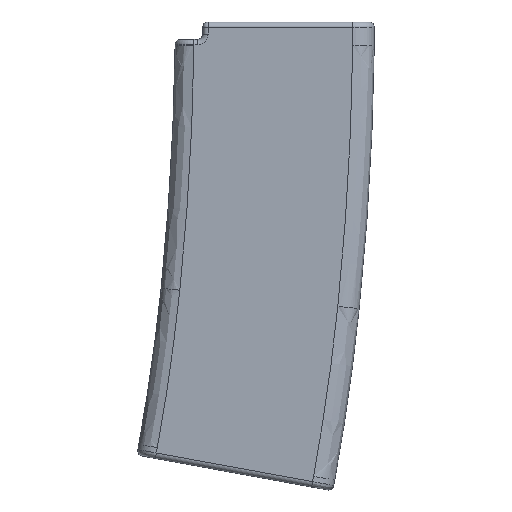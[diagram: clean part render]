
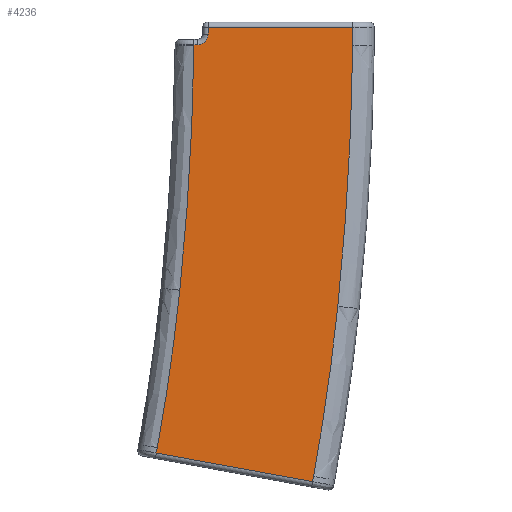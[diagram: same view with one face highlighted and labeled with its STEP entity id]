
A CAD part, top view. The second image highlights one B-rep face of the part: STEP entity #4236.
In plain terms, the highlighted planar face has unit normal (0, 0, 1).
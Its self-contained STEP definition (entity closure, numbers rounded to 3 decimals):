
#112=PLANE('',#4756);
#263=LINE('',#8074,#506);
#296=LINE('',#8319,#539);
#298=LINE('',#8379,#541);
#300=LINE('',#8392,#543);
#302=LINE('',#8400,#545);
#321=LINE('',#8475,#564);
#349=LINE('',#9411,#592);
#352=LINE('',#9417,#595);
#506=VECTOR('',#5561,10.);
#539=VECTOR('',#5660,10.);
#541=VECTOR('',#5662,10.);
#543=VECTOR('',#5678,10.);
#545=VECTOR('',#5686,10.);
#564=VECTOR('',#5777,10.);
#592=VECTOR('',#5985,10.);
#595=VECTOR('',#5994,10.);
#1068=FACE_OUTER_BOUND('',#1337,.T.);
#1337=EDGE_LOOP('',(#3874,#3875,#3876,#3877,#3878,#3879,#3880,#3881,#3882,
#3883,#3884,#3885,#3886));
#1572=CIRCLE('',#4622,4.);
#1610=CIRCLE('',#4688,758.056);
#1611=CIRCLE('',#4689,817.052);
#1641=CIRCLE('',#4727,1007.674);
#1643=CIRCLE('',#4729,1066.669);
#1935=VERTEX_POINT('',#8063);
#1936=VERTEX_POINT('',#8072);
#1957=VERTEX_POINT('',#8318);
#1959=VERTEX_POINT('',#8362);
#1960=VERTEX_POINT('',#8383);
#1962=VERTEX_POINT('',#8387);
#1963=VERTEX_POINT('',#8391);
#1966=VERTEX_POINT('',#8399);
#1986=VERTEX_POINT('',#8473);
#2001=VERTEX_POINT('',#8951);
#2003=VERTEX_POINT('',#9006);
#2013=VERTEX_POINT('',#9330);
#2015=VERTEX_POINT('',#9343);
#2451=EDGE_CURVE('',#1935,#1936,#263,.T.);
#2499=EDGE_CURVE('',#1957,#1936,#296,.T.);
#2503=EDGE_CURVE('',#1959,#1935,#298,.T.);
#2508=EDGE_CURVE('',#1962,#1960,#1572,.T.);
#2509=EDGE_CURVE('',#1960,#1963,#300,.T.);
#2513=EDGE_CURVE('',#1963,#1966,#302,.T.);
#2552=EDGE_CURVE('',#1986,#1962,#321,.T.);
#2587=EDGE_CURVE('',#2001,#1957,#1610,.T.);
#2589=EDGE_CURVE('',#2003,#1959,#1611,.T.);
#2625=EDGE_CURVE('',#2013,#2001,#1641,.T.);
#2627=EDGE_CURVE('',#2015,#2003,#1643,.T.);
#2652=EDGE_CURVE('',#1986,#2013,#349,.T.);
#2655=EDGE_CURVE('',#2015,#1966,#352,.T.);
#3874=ORIENTED_EDGE('',*,*,#2451,.F.);
#3875=ORIENTED_EDGE('',*,*,#2503,.F.);
#3876=ORIENTED_EDGE('',*,*,#2589,.F.);
#3877=ORIENTED_EDGE('',*,*,#2627,.F.);
#3878=ORIENTED_EDGE('',*,*,#2655,.T.);
#3879=ORIENTED_EDGE('',*,*,#2513,.F.);
#3880=ORIENTED_EDGE('',*,*,#2509,.F.);
#3881=ORIENTED_EDGE('',*,*,#2508,.F.);
#3882=ORIENTED_EDGE('',*,*,#2552,.F.);
#3883=ORIENTED_EDGE('',*,*,#2652,.T.);
#3884=ORIENTED_EDGE('',*,*,#2625,.T.);
#3885=ORIENTED_EDGE('',*,*,#2587,.T.);
#3886=ORIENTED_EDGE('',*,*,#2499,.T.);
#4236=ADVANCED_FACE('',(#1068),#112,.T.);
#4622=AXIS2_PLACEMENT_3D('',#8389,#5674,#5675);
#4688=AXIS2_PLACEMENT_3D('',#8968,#5836,#5837);
#4689=AXIS2_PLACEMENT_3D('',#9023,#5838,#5839);
#4727=AXIS2_PLACEMENT_3D('',#9332,#5918,#5919);
#4729=AXIS2_PLACEMENT_3D('',#9345,#5922,#5923);
#4756=AXIS2_PLACEMENT_3D('',#9418,#5995,#5996);
#5561=DIRECTION('',(-0.984,0.18,0.));
#5660=DIRECTION('',(-0.18,-0.984,0.));
#5662=DIRECTION('',(-0.18,-0.984,0.));
#5674=DIRECTION('center_axis',(0.,0.,1.));
#5675=DIRECTION('ref_axis',(0.487,-0.873,0.));
#5678=DIRECTION('',(0.,1.,0.));
#5686=DIRECTION('',(1.,0.,0.));
#5777=DIRECTION('',(1.,0.,0.));
#5836=DIRECTION('center_axis',(0.,0.,-1.));
#5837=DIRECTION('ref_axis',(0.995,-0.103,0.));
#5838=DIRECTION('center_axis',(0.,0.,-1.));
#5839=DIRECTION('ref_axis',(0.995,-0.103,0.));
#5918=DIRECTION('center_axis',(0.,0.,
-1.));
#5919=DIRECTION('ref_axis',(1.,-0.013,0.));
#5922=DIRECTION('center_axis',(0.,0.,
-1.));
#5923=DIRECTION('ref_axis',(1.,-0.012,0.));
#5985=DIRECTION('',(0.,-1.,0.));
#5994=DIRECTION('',(0.,1.,0.));
#5995=DIRECTION('center_axis',(0.,0.,1.));
#5996=DIRECTION('ref_axis',(1.,0.,0.));
#8063=CARTESIAN_POINT('',(9.817,-164.25,14.95));
#8072=CARTESIAN_POINT('',(-48.216,-153.638,14.95));
#8074=CARTESIAN_POINT('',(-38.643,-155.388,14.95));
#8318=CARTESIAN_POINT('',(-47.856,-151.67,14.95));
#8319=CARTESIAN_POINT('',(-47.856,-151.67,14.95));
#8362=CARTESIAN_POINT('',(10.177,-162.283,14.95));
#8379=CARTESIAN_POINT('',(10.177,-162.283,14.95));
#8383=CARTESIAN_POINT('',(-29.,2.,14.95));
#8387=CARTESIAN_POINT('',(-33.,-2.,14.95));
#8389=CARTESIAN_POINT('Origin',(-33.,2.,14.95));
#8391=CARTESIAN_POINT('',(-29.,4.5,14.95));
#8392=CARTESIAN_POINT('',(-29.,-1.15,14.95));
#8399=CARTESIAN_POINT('',(24.75,4.5,14.95));
#8400=CARTESIAN_POINT('',(-15.625,4.5,14.95));
#8473=CARTESIAN_POINT('',(-34.25,-2.,14.95));
#8475=CARTESIAN_POINT('',(-16.875,-2.,14.95));
#8951=CARTESIAN_POINT('',(-39.497,-93.128,14.95));
#8968=CARTESIAN_POINT('Origin',(-793.549,-15.321,14.95));
#9006=CARTESIAN_POINT('',(19.187,-99.184,14.95));
#9023=CARTESIAN_POINT('Origin',(-793.549,-15.321,14.95));
#9330=CARTESIAN_POINT('',(-34.25,-2.3,14.95));
#9332=CARTESIAN_POINT('Origin',(-1041.844,10.336,14.95));
#9343=CARTESIAN_POINT('',(24.75,-2.3,14.95));
#9345=CARTESIAN_POINT('Origin',(-1041.844,10.336,14.95));
#9411=CARTESIAN_POINT('',(-34.25,0.,14.95));
#9417=CARTESIAN_POINT('',(24.75,-2.3,14.95));
#9418=CARTESIAN_POINT('Origin',(-31.25,-2.3,14.95));
